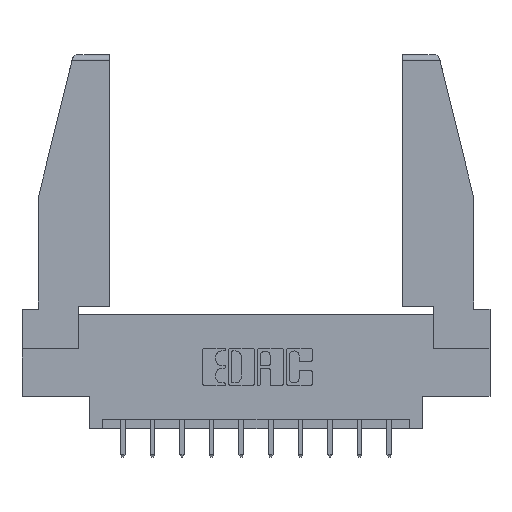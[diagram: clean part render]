
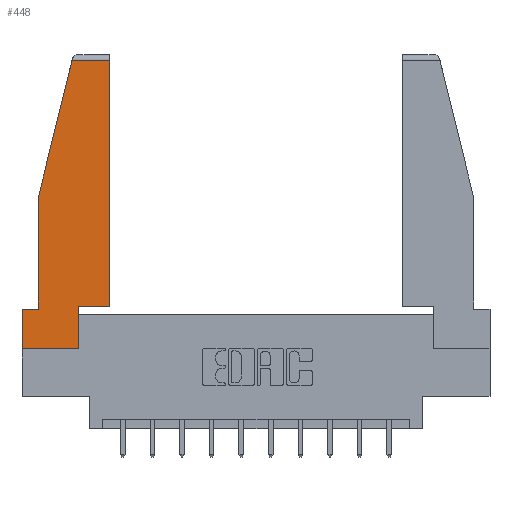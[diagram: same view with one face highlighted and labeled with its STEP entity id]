
A CAD part, top view. The second image highlights one B-rep face of the part: STEP entity #448.
In plain terms, the highlighted planar face has unit normal (0, 0, 1).
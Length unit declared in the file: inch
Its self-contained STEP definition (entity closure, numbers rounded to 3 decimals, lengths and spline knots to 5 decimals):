
#164 = DIRECTION ( 'NONE',  ( 0., 1., 0. ) ) ;
#325 = CARTESIAN_POINT ( 'NONE',  ( 0., 0.21, 0. ) ) ;
#448 = ADVANCED_FACE ( 'NONE', ( #13659 ), #6852, .T. ) ;
#661 = VERTEX_POINT ( 'NONE', #3334 ) ;
#855 = ORIENTED_EDGE ( 'NONE', *, *, #6906, .T. ) ;
#937 = CARTESIAN_POINT ( 'NONE',  ( 0.297, 0., 0. ) ) ;
#1224 = VECTOR ( 'NONE', #9048, 39.37008 ) ;
#1236 = CARTESIAN_POINT ( 'NONE',  ( 0., 0., 0. ) ) ;
#1401 = LINE ( 'NONE', #7506, #7538 ) ;
#1539 = DIRECTION ( 'NONE',  ( 1., 0., 0. ) ) ;
#1785 = VECTOR ( 'NONE', #7133, 39.37008 ) ;
#2251 = CARTESIAN_POINT ( 'NONE',  ( 0.271, 1.55, 0. ) ) ;
#2304 = DIRECTION ( 'NONE',  ( 0., 0., 1. ) ) ;
#2406 = CARTESIAN_POINT ( 'NONE',  ( 0., 0., 0. ) ) ;
#2483 = VECTOR ( 'NONE', #4634, 39.37008 ) ;
#2637 = CARTESIAN_POINT ( 'NONE',  ( 0.461, 0.223, 0. ) ) ;
#2651 = CARTESIAN_POINT ( 'NONE',  ( 0.297, 0.223, 0. ) ) ;
#2671 = CARTESIAN_POINT ( 'NONE',  ( 0., 0.21, 0. ) ) ;
#2711 = VERTEX_POINT ( 'NONE', #3419 ) ;
#2851 = DIRECTION ( 'NONE',  ( -1., 0., 0. ) ) ;
#2893 = ORIENTED_EDGE ( 'NONE', *, *, #5130, .T. ) ;
#2979 = VECTOR ( 'NONE', #2851, 39.37008 ) ;
#3334 = CARTESIAN_POINT ( 'NONE',  ( 0.297, 0.223, 0. ) ) ;
#3375 = VERTEX_POINT ( 'NONE', #9549 ) ;
#3419 = CARTESIAN_POINT ( 'NONE',  ( 0.461, 1.52, 0. ) ) ;
#3494 = VECTOR ( 'NONE', #1539, 39.37008 ) ;
#3591 = LINE ( 'NONE', #325, #8481 ) ;
#3800 = VERTEX_POINT ( 'NONE', #2406 ) ;
#4158 = VERTEX_POINT ( 'NONE', #937 ) ;
#4164 = VERTEX_POINT ( 'NONE', #14402 ) ;
#4232 = CARTESIAN_POINT ( 'NONE',  ( 0.297, 0., 0. ) ) ;
#4634 = DIRECTION ( 'NONE',  ( -0.239, -0.971, 0. ) ) ;
#4726 = EDGE_CURVE ( 'NONE', #2711, #4164, #7555, .T. ) ;
#4749 = EDGE_CURVE ( 'NONE', #661, #7522, #6499, .T. ) ;
#4890 = LINE ( 'NONE', #1236, #1224 ) ;
#4952 = ORIENTED_EDGE ( 'NONE', *, *, #12432, .T. ) ;
#5130 = EDGE_CURVE ( 'NONE', #3800, #4158, #4890, .T. ) ;
#5282 = LINE ( 'NONE', #2671, #1785 ) ;
#6128 = ORIENTED_EDGE ( 'NONE', *, *, #4726, .T. ) ;
#6223 = VECTOR ( 'NONE', #9750, 39.37008 ) ;
#6453 = VERTEX_POINT ( 'NONE', #8575 ) ;
#6499 = LINE ( 'NONE', #2651, #3494 ) ;
#6506 = ORIENTED_EDGE ( 'NONE', *, *, #9265, .T. ) ;
#6852 = PLANE ( 'NONE',  #11378 ) ;
#6906 = EDGE_CURVE ( 'NONE', #6453, #9387, #3591, .T. ) ;
#6978 = ORIENTED_EDGE ( 'NONE', *, *, #4749, .T. ) ;
#7001 = LINE ( 'NONE', #11267, #9263 ) ;
#7133 = DIRECTION ( 'NONE',  ( 0., -1., 0. ) ) ;
#7506 = CARTESIAN_POINT ( 'NONE',  ( 0.086, 0.8, 0. ) ) ;
#7522 = VERTEX_POINT ( 'NONE', #2637 ) ;
#7538 = VECTOR ( 'NONE', #8554, 39.37008 ) ;
#7555 = LINE ( 'NONE', #13967, #2979 ) ;
#7766 = EDGE_CURVE ( 'NONE', #4158, #661, #10961, .T. ) ;
#8481 = VECTOR ( 'NONE', #13965, 39.37008 ) ;
#8554 = DIRECTION ( 'NONE',  ( 0., -1., 0. ) ) ;
#8575 = CARTESIAN_POINT ( 'NONE',  ( 0.086, 0.21, 0. ) ) ;
#9048 = DIRECTION ( 'NONE',  ( 1., 0., 0. ) ) ;
#9126 = LINE ( 'NONE', #2251, #2483 ) ;
#9263 = VECTOR ( 'NONE', #164, 39.37008 ) ;
#9265 = EDGE_CURVE ( 'NONE', #4164, #3375, #9126, .T. ) ;
#9354 = EDGE_CURVE ( 'NONE', #9387, #3800, #5282, .T. ) ;
#9387 = VERTEX_POINT ( 'NONE', #12323 ) ;
#9549 = CARTESIAN_POINT ( 'NONE',  ( 0.086, 0.8, 0. ) ) ;
#9750 = DIRECTION ( 'NONE',  ( 0., 1., 0. ) ) ;
#10112 = CARTESIAN_POINT ( 'NONE',  ( 0., 0., 0. ) ) ;
#10302 = ORIENTED_EDGE ( 'NONE', *, *, #7766, .T. ) ;
#10616 = EDGE_LOOP ( 'NONE', ( #4952, #6128, #6506, #12151, #855, #13872, #2893, #10302, #6978 ) ) ;
#10961 = LINE ( 'NONE', #4232, #6223 ) ;
#11267 = CARTESIAN_POINT ( 'NONE',  ( 0.461, 0.223, 0. ) ) ;
#11306 = DIRECTION ( 'NONE',  ( 1., 0., 0. ) ) ;
#11378 = AXIS2_PLACEMENT_3D ( 'NONE', #10112, #2304, #11306 ) ;
#11389 = EDGE_CURVE ( 'NONE', #3375, #6453, #1401, .T. ) ;
#12151 = ORIENTED_EDGE ( 'NONE', *, *, #11389, .T. ) ;
#12323 = CARTESIAN_POINT ( 'NONE',  ( 0., 0.21, 0. ) ) ;
#12432 = EDGE_CURVE ( 'NONE', #7522, #2711, #7001, .T. ) ;
#13659 = FACE_OUTER_BOUND ( 'NONE', #10616, .T. ) ;
#13872 = ORIENTED_EDGE ( 'NONE', *, *, #9354, .T. ) ;
#13965 = DIRECTION ( 'NONE',  ( -1., 0., 0. ) ) ;
#13967 = CARTESIAN_POINT ( 'NONE',  ( 0., 1.52, 0. ) ) ;
#14402 = CARTESIAN_POINT ( 'NONE',  ( 0.2636, 1.52, 0. ) ) ;
